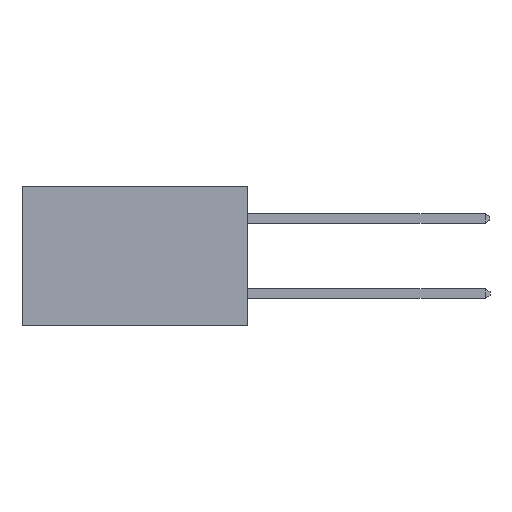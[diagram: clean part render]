
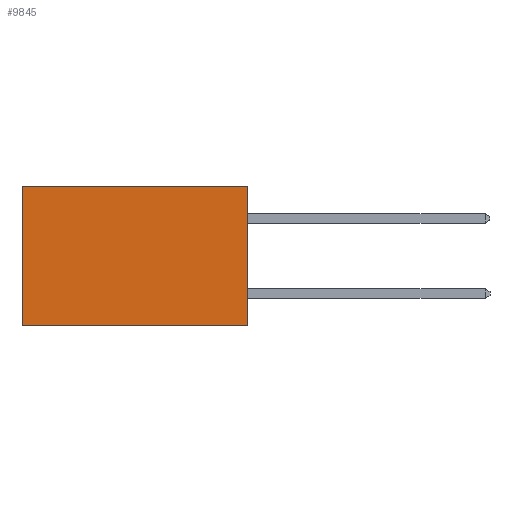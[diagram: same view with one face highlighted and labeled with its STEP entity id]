
A CAD part, left-side view. The second image highlights one B-rep face of the part: STEP entity #9845.
In plain terms, the highlighted planar face has unit normal (-1, 0, 0).
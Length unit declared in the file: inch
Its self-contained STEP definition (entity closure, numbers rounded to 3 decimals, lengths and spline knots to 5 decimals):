
#338 = DIRECTION ( 'NONE',  ( 0., 0., -1. ) ) ;
#731 = CARTESIAN_POINT ( 'NONE',  ( 0.2615, 0., -0.37 ) ) ;
#817 = CARTESIAN_POINT ( 'NONE',  ( 0.2615, 0.6, -0.37 ) ) ;
#1428 = FACE_OUTER_BOUND ( 'NONE', #11423, .T. ) ;
#1821 = DIRECTION ( 'NONE',  ( 0., 1., 0. ) ) ;
#1862 = CARTESIAN_POINT ( 'NONE',  ( 0.2615, 0., -0.37 ) ) ;
#2167 = AXIS2_PLACEMENT_3D ( 'NONE', #2434, #5410, #5176 ) ;
#2406 = EDGE_CURVE ( 'NONE', #4844, #6442, #6727, .T. ) ;
#2434 = CARTESIAN_POINT ( 'NONE',  ( 0.2615, 0., -0.37 ) ) ;
#2644 = CARTESIAN_POINT ( 'NONE',  ( 0.2615, 0., 0. ) ) ;
#2807 = CARTESIAN_POINT ( 'NONE',  ( 0.2615, 0.6, 0. ) ) ;
#3198 = DIRECTION ( 'NONE',  ( 0., 1., 0. ) ) ;
#3534 = PLANE ( 'NONE',  #2167 ) ;
#3682 = VECTOR ( 'NONE', #7883, 39.37008 ) ;
#3951 = LINE ( 'NONE', #7894, #3682 ) ;
#4318 = LINE ( 'NONE', #2644, #6762 ) ;
#4681 = CARTESIAN_POINT ( 'NONE',  ( 0.2615, 0., -0.37 ) ) ;
#4844 = VERTEX_POINT ( 'NONE', #4681 ) ;
#5176 = DIRECTION ( 'NONE',  ( 0., 0., -1. ) ) ;
#5410 = DIRECTION ( 'NONE',  ( 1., 0., 0. ) ) ;
#5970 = EDGE_CURVE ( 'NONE', #10240, #4844, #8794, .T. ) ;
#6372 = VECTOR ( 'NONE', #338, 39.37008 ) ;
#6442 = VERTEX_POINT ( 'NONE', #817 ) ;
#6727 = LINE ( 'NONE', #1862, #11458 ) ;
#6762 = VECTOR ( 'NONE', #3198, 39.37008 ) ;
#7057 = ORIENTED_EDGE ( 'NONE', *, *, #2406, .F. ) ;
#7372 = ORIENTED_EDGE ( 'NONE', *, *, #11591, .T. ) ;
#7883 = DIRECTION ( 'NONE',  ( 0., 0., -1. ) ) ;
#7894 = CARTESIAN_POINT ( 'NONE',  ( 0.2615, 0.6, -0.37 ) ) ;
#7946 = ORIENTED_EDGE ( 'NONE', *, *, #5970, .F. ) ;
#8077 = ORIENTED_EDGE ( 'NONE', *, *, #8906, .T. ) ;
#8406 = CARTESIAN_POINT ( 'NONE',  ( 0.2615, 0., 0. ) ) ;
#8518 = VERTEX_POINT ( 'NONE', #2807 ) ;
#8794 = LINE ( 'NONE', #731, #6372 ) ;
#8906 = EDGE_CURVE ( 'NONE', #8518, #6442, #3951, .T. ) ;
#9845 = ADVANCED_FACE ( 'NONE', ( #1428 ), #3534, .F. ) ;
#10240 = VERTEX_POINT ( 'NONE', #8406 ) ;
#11423 = EDGE_LOOP ( 'NONE', ( #8077, #7057, #7946, #7372 ) ) ;
#11458 = VECTOR ( 'NONE', #1821, 39.37008 ) ;
#11591 = EDGE_CURVE ( 'NONE', #10240, #8518, #4318, .T. ) ;
